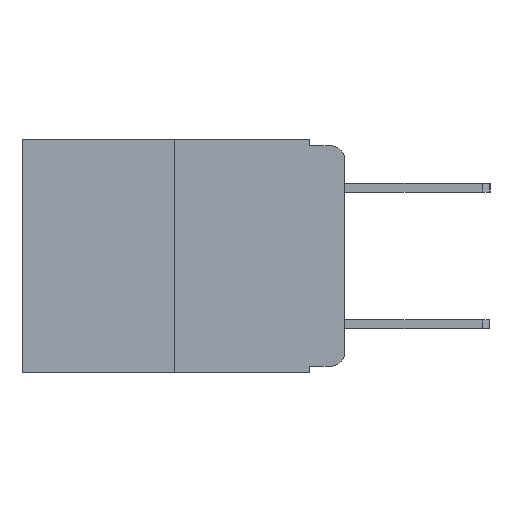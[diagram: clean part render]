
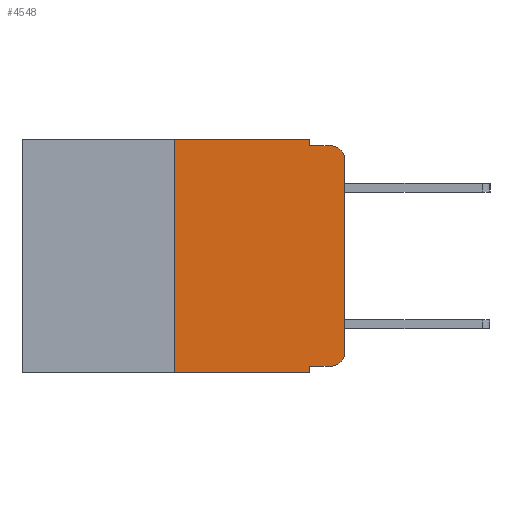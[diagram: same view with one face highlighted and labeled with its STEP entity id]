
A CAD part, left-side view. The second image highlights one B-rep face of the part: STEP entity #4548.
In plain terms, the highlighted planar face has unit normal (-1, 0, 0).
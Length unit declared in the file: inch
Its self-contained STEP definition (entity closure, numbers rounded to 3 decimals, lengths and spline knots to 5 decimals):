
#524 = EDGE_CURVE ( 'NONE', #5944, #8381, #8655, .T. ) ;
#832 = ORIENTED_EDGE ( 'NONE', *, *, #2060, .T. ) ;
#1307 = EDGE_CURVE ( 'NONE', #8381, #9361, #11665, .T. ) ;
#1308 = CARTESIAN_POINT ( 'NONE',  ( 0., 0., 0. ) ) ;
#1323 = DIRECTION ( 'NONE',  ( 0., 0., 1. ) ) ;
#1441 = VECTOR ( 'NONE', #12210, 39.37008 ) ;
#1712 = CARTESIAN_POINT ( 'NONE',  ( 0., 0.473, 0. ) ) ;
#1811 = VECTOR ( 'NONE', #3929, 39.37008 ) ;
#2060 = EDGE_CURVE ( 'NONE', #6148, #9361, #4004, .T. ) ;
#2101 = AXIS2_PLACEMENT_3D ( 'NONE', #8826, #8742, #8774 ) ;
#2316 = VERTEX_POINT ( 'NONE', #5334 ) ;
#2639 = LINE ( 'NONE', #12516, #12617 ) ;
#2770 = EDGE_CURVE ( 'NONE', #12513, #6148, #8001, .T. ) ;
#2799 = DIRECTION ( 'NONE',  ( 0., 0., -1. ) ) ;
#2910 = CARTESIAN_POINT ( 'NONE',  ( 0., 0.051, 0. ) ) ;
#3310 = VECTOR ( 'NONE', #7474, 39.37008 ) ;
#3348 = VECTOR ( 'NONE', #11295, 39.37008 ) ;
#3362 = CARTESIAN_POINT ( 'NONE',  ( 0., 0.25, 0. ) ) ;
#3589 = VERTEX_POINT ( 'NONE', #7138 ) ;
#3929 = DIRECTION ( 'NONE',  ( 0., -1., 0. ) ) ;
#4004 = CIRCLE ( 'NONE', #2101, 0.02 ) ;
#4081 = ORIENTED_EDGE ( 'NONE', *, *, #12699, .F. ) ;
#4333 = CARTESIAN_POINT ( 'NONE',  ( 0., 0.473, 0. ) ) ;
#4542 = ORIENTED_EDGE ( 'NONE', *, *, #10937, .T. ) ;
#4548 = ADVANCED_FACE ( 'NONE', ( #6758 ), #7778, .F. ) ;
#4843 = VERTEX_POINT ( 'NONE', #3362 ) ;
#4935 = CARTESIAN_POINT ( 'NONE',  ( 0., 0.051, -0.01 ) ) ;
#5131 = DIRECTION ( 'NONE',  ( -1., 0., 0. ) ) ;
#5183 = CARTESIAN_POINT ( 'NONE',  ( 0., 0.25, -0.343 ) ) ;
#5219 = EDGE_CURVE ( 'NONE', #4843, #5944, #8261, .T. ) ;
#5255 = VERTEX_POINT ( 'NONE', #11994 ) ;
#5300 = CARTESIAN_POINT ( 'NONE',  ( 0., 0.02, -0.01 ) ) ;
#5316 = CARTESIAN_POINT ( 'NONE',  ( 0., 0.051, 0. ) ) ;
#5334 = CARTESIAN_POINT ( 'NONE',  ( 0., 0.051, -0.333 ) ) ;
#5944 = VERTEX_POINT ( 'NONE', #5316 ) ;
#6148 = VERTEX_POINT ( 'NONE', #12276 ) ;
#6396 = ORIENTED_EDGE ( 'NONE', *, *, #1307, .F. ) ;
#6685 = AXIS2_PLACEMENT_3D ( 'NONE', #10902, #5131, #11797 ) ;
#6708 = ORIENTED_EDGE ( 'NONE', *, *, #11697, .T. ) ;
#6758 = FACE_OUTER_BOUND ( 'NONE', #7406, .T. ) ;
#6875 = CARTESIAN_POINT ( 'NONE',  ( 0., 0.051, -0.333 ) ) ;
#7019 = ORIENTED_EDGE ( 'NONE', *, *, #12115, .F. ) ;
#7077 = VECTOR ( 'NONE', #1323, 39.37008 ) ;
#7138 = CARTESIAN_POINT ( 'NONE',  ( 0., 0.051, -0.343 ) ) ;
#7244 = VECTOR ( 'NONE', #11033, 39.37008 ) ;
#7406 = EDGE_LOOP ( 'NONE', ( #11171, #832, #6396, #9015, #11450, #4081, #6708, #7019, #9577, #4542 ) ) ;
#7444 = CARTESIAN_POINT ( 'NONE',  ( 0., 0.051, -0.01 ) ) ;
#7474 = DIRECTION ( 'NONE',  ( 0., 0., -1. ) ) ;
#7778 = PLANE ( 'NONE',  #9199 ) ;
#7891 = CIRCLE ( 'NONE', #6685, 0.02 ) ;
#7941 = VERTEX_POINT ( 'NONE', #5183 ) ;
#8001 = LINE ( 'NONE', #1308, #7077 ) ;
#8239 = CARTESIAN_POINT ( 'NONE',  ( 0., 0.25, 0. ) ) ;
#8261 = LINE ( 'NONE', #4333, #10779 ) ;
#8381 = VERTEX_POINT ( 'NONE', #4935 ) ;
#8482 = CARTESIAN_POINT ( 'NONE',  ( 0., 0.051, 0. ) ) ;
#8615 = LINE ( 'NONE', #8482, #3310 ) ;
#8655 = LINE ( 'NONE', #2910, #3348 ) ;
#8742 = DIRECTION ( 'NONE',  ( -1., 0., 0. ) ) ;
#8774 = DIRECTION ( 'NONE',  ( 0., 0., -1. ) ) ;
#8818 = DIRECTION ( 'NONE',  ( 1., 0., 0. ) ) ;
#8826 = CARTESIAN_POINT ( 'NONE',  ( 0., 0.02, -0.03 ) ) ;
#8945 = CARTESIAN_POINT ( 'NONE',  ( 0., 0., -0.313 ) ) ;
#9015 = ORIENTED_EDGE ( 'NONE', *, *, #524, .F. ) ;
#9196 = DIRECTION ( 'NONE',  ( 0., -1., 0. ) ) ;
#9199 = AXIS2_PLACEMENT_3D ( 'NONE', #1712, #8818, #2799 ) ;
#9361 = VERTEX_POINT ( 'NONE', #5300 ) ;
#9577 = ORIENTED_EDGE ( 'NONE', *, *, #11536, .T. ) ;
#9795 = LINE ( 'NONE', #8239, #7244 ) ;
#9806 = LINE ( 'NONE', #6875, #1811 ) ;
#9839 = DIRECTION ( 'NONE',  ( 0., -1., 0. ) ) ;
#10779 = VECTOR ( 'NONE', #9196, 39.37008 ) ;
#10902 = CARTESIAN_POINT ( 'NONE',  ( 0., 0.02, -0.313 ) ) ;
#10937 = EDGE_CURVE ( 'NONE', #5255, #12513, #7891, .T. ) ;
#11033 = DIRECTION ( 'NONE',  ( 0., 0., 1. ) ) ;
#11171 = ORIENTED_EDGE ( 'NONE', *, *, #2770, .T. ) ;
#11295 = DIRECTION ( 'NONE',  ( 0., 0., -1. ) ) ;
#11450 = ORIENTED_EDGE ( 'NONE', *, *, #5219, .F. ) ;
#11536 = EDGE_CURVE ( 'NONE', #2316, #5255, #9806, .T. ) ;
#11665 = LINE ( 'NONE', #7444, #1441 ) ;
#11697 = EDGE_CURVE ( 'NONE', #7941, #3589, #2639, .T. ) ;
#11797 = DIRECTION ( 'NONE',  ( 0., 0., -1. ) ) ;
#11994 = CARTESIAN_POINT ( 'NONE',  ( 0., 0.02, -0.333 ) ) ;
#12115 = EDGE_CURVE ( 'NONE', #2316, #3589, #8615, .T. ) ;
#12210 = DIRECTION ( 'NONE',  ( 0., -1., 0. ) ) ;
#12276 = CARTESIAN_POINT ( 'NONE',  ( 0., 0., -0.03 ) ) ;
#12513 = VERTEX_POINT ( 'NONE', #8945 ) ;
#12516 = CARTESIAN_POINT ( 'NONE',  ( 0., 0.473, -0.343 ) ) ;
#12617 = VECTOR ( 'NONE', #9839, 39.37008 ) ;
#12699 = EDGE_CURVE ( 'NONE', #7941, #4843, #9795, .T. ) ;
